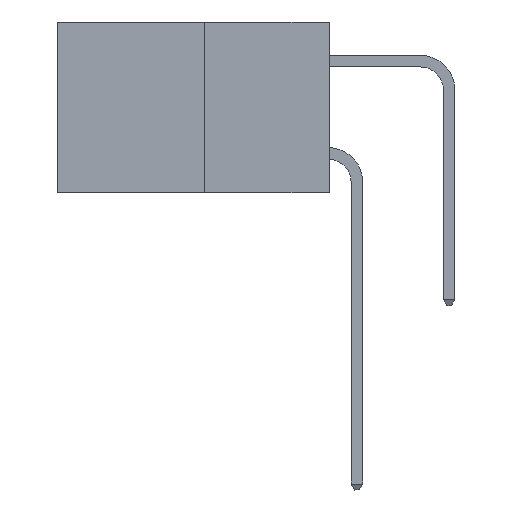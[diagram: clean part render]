
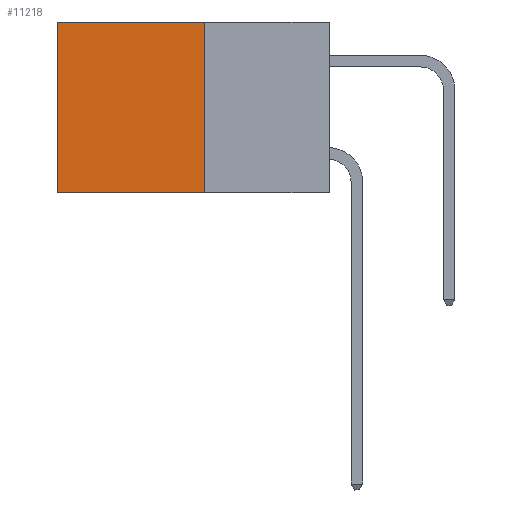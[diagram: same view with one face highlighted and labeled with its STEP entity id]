
A CAD part, left-side view. The second image highlights one B-rep face of the part: STEP entity #11218.
In plain terms, the highlighted planar face has unit normal (-1, 0, 0).
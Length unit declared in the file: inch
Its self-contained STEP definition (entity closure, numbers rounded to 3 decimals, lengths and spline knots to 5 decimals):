
#750 = CARTESIAN_POINT ( 'NONE',  ( 0.277, 0.27, -0.37 ) ) ;
#868 = CARTESIAN_POINT ( 'NONE',  ( 0.277, 0.59, 0. ) ) ;
#3029 = EDGE_CURVE ( 'NONE', #3970, #15469, #3525, .T. ) ;
#3191 = VECTOR ( 'NONE', #12938, 39.37008 ) ;
#3525 = LINE ( 'NONE', #12455, #12294 ) ;
#3970 = VERTEX_POINT ( 'NONE', #6192 ) ;
#5124 = CARTESIAN_POINT ( 'NONE',  ( 0.277, 0.59, -0.37 ) ) ;
#5574 = VERTEX_POINT ( 'NONE', #12026 ) ;
#6192 = CARTESIAN_POINT ( 'NONE',  ( 0.277, 0.27, 0. ) ) ;
#6923 = ORIENTED_EDGE ( 'NONE', *, *, #20644, .F. ) ;
#7353 = LINE ( 'NONE', #7796, #3191 ) ;
#7515 = ORIENTED_EDGE ( 'NONE', *, *, #3029, .T. ) ;
#7682 = DIRECTION ( 'NONE',  ( 0., 1., 0. ) ) ;
#7796 = CARTESIAN_POINT ( 'NONE',  ( 0.277, 0.27, -0.37 ) ) ;
#7836 = DIRECTION ( 'NONE',  ( 0., 0., -1. ) ) ;
#7840 = EDGE_LOOP ( 'NONE', ( #9743, #6923, #14946, #7515 ) ) ;
#8341 = EDGE_CURVE ( 'NONE', #15469, #13742, #12309, .T. ) ;
#9743 = ORIENTED_EDGE ( 'NONE', *, *, #8341, .T. ) ;
#11065 = CARTESIAN_POINT ( 'NONE',  ( 0.277, 0.27, -0.37 ) ) ;
#11218 = ADVANCED_FACE ( 'NONE', ( #21116 ), #16427, .F. ) ;
#12022 = CARTESIAN_POINT ( 'NONE',  ( 0.277, 0.59, -0.37 ) ) ;
#12026 = CARTESIAN_POINT ( 'NONE',  ( 0.277, 0.27, -0.37 ) ) ;
#12237 = DIRECTION ( 'NONE',  ( 0., 1., 0. ) ) ;
#12294 = VECTOR ( 'NONE', #12237, 39.37008 ) ;
#12309 = LINE ( 'NONE', #12022, #20199 ) ;
#12317 = DIRECTION ( 'NONE',  ( 0., 0., -1. ) ) ;
#12455 = CARTESIAN_POINT ( 'NONE',  ( 0.277, 0.27, 0. ) ) ;
#12938 = DIRECTION ( 'NONE',  ( 0., 0., -1. ) ) ;
#13742 = VERTEX_POINT ( 'NONE', #5124 ) ;
#14946 = ORIENTED_EDGE ( 'NONE', *, *, #21320, .F. ) ;
#15469 = VERTEX_POINT ( 'NONE', #868 ) ;
#16427 = PLANE ( 'NONE',  #21565 ) ;
#18084 = DIRECTION ( 'NONE',  ( 1., 0., 0. ) ) ;
#20199 = VECTOR ( 'NONE', #12317, 39.37008 ) ;
#20644 = EDGE_CURVE ( 'NONE', #5574, #13742, #21410, .T. ) ;
#21116 = FACE_OUTER_BOUND ( 'NONE', #7840, .T. ) ;
#21177 = VECTOR ( 'NONE', #7682, 39.37008 ) ;
#21320 = EDGE_CURVE ( 'NONE', #3970, #5574, #7353, .T. ) ;
#21410 = LINE ( 'NONE', #11065, #21177 ) ;
#21565 = AXIS2_PLACEMENT_3D ( 'NONE', #750, #18084, #7836 ) ;
